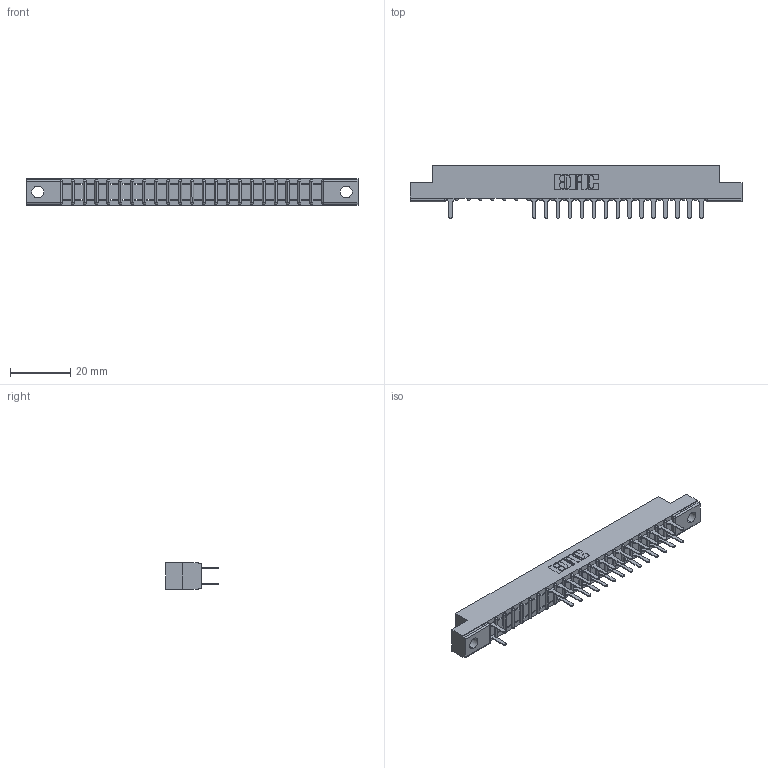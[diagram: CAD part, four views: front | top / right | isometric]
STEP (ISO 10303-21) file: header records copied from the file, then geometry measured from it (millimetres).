
FILE_DESCRIPTION (( 'STEP AP203' ), '1' );
FILE_NAME ('307-044-520-204.STEP', '2018-08-06T02:13:24', ( '' ), ( '' ), 'SwSTEP 2.0', 'SolidWorks 2016', '' );
FILE_SCHEMA (( 'CONFIG_CONTROL_DESIGN' ));
Length unit declared in the file: inch
Products named in the file (3): 307 Part_.156 Dia Mounting Holes; 307-290-001_520; 307-044-520-204
Assembly tree (32 placements, depth 2):
  307-044-520-204
    307 Part_.156 Dia Mounting Holes
    307-290-001_520  x31
Bounding box: 110.19 x 17.42 x 8.71 mm (x, y, z)
Volume: 6955.7 mm3; surface area: 11265.1 mm2
Topology: 32 solids, 32 shells, 1711 faces, 4805 edges, 3098 vertices
Faces by surface type: plane 1123, cylinder 542, sphere 46
Entity records: 22000 total; most frequent: CARTESIAN_POINT 3663, ORIENTED_EDGE 3638, DIRECTION 3575, EDGE_CURVE 1819, VECTOR 1395, LINE 1395, VERTEX_POINT 1178, AXIS2_PLACEMENT_3D 1090
